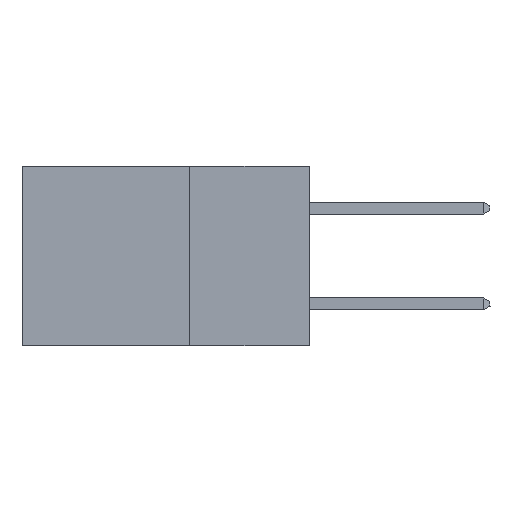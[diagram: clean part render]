
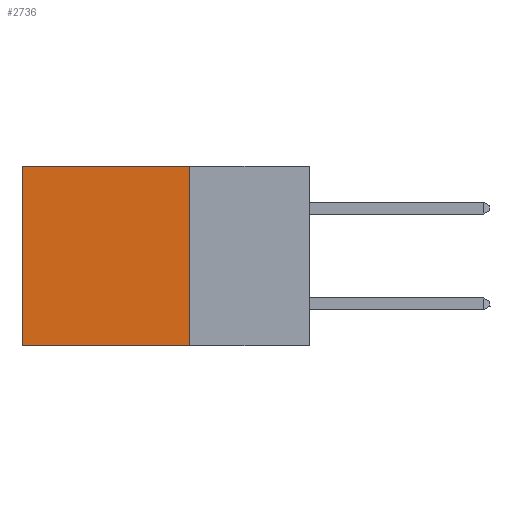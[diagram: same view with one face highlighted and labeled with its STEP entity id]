
A CAD part, left-side view. The second image highlights one B-rep face of the part: STEP entity #2736.
In plain terms, the highlighted planar face has unit normal (-1, 0, 0).
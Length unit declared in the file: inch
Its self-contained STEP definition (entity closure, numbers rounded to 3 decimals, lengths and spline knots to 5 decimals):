
#719 = ORIENTED_EDGE ( 'NONE', *, *, #4456, .T. ) ;
#1037 = EDGE_CURVE ( 'NONE', #16225, #10508, #19683, .T. ) ;
#1660 = VECTOR ( 'NONE', #12428, 39.37008 ) ;
#1872 = LINE ( 'NONE', #16064, #6905 ) ;
#2736 = ADVANCED_FACE ( 'NONE', ( #14826 ), #18105, .F. ) ;
#4456 = EDGE_CURVE ( 'NONE', #16225, #9502, #1872, .T. ) ;
#5193 = DIRECTION ( 'NONE',  ( 0., 1., 0. ) ) ;
#5533 = LINE ( 'NONE', #5628, #10541 ) ;
#5628 = CARTESIAN_POINT ( 'NONE',  ( 0.2875, 0.6, -0.375 ) ) ;
#6150 = EDGE_CURVE ( 'NONE', #9502, #11161, #5533, .T. ) ;
#6254 = ORIENTED_EDGE ( 'NONE', *, *, #1037, .F. ) ;
#6905 = VECTOR ( 'NONE', #20877, 39.37008 ) ;
#7322 = DIRECTION ( 'NONE',  ( 0., 0., -1. ) ) ;
#9097 = CARTESIAN_POINT ( 'NONE',  ( 0.2875, 0.25, 0. ) ) ;
#9502 = VERTEX_POINT ( 'NONE', #19865 ) ;
#9515 = DIRECTION ( 'NONE',  ( 0., 0., -1. ) ) ;
#10508 = VERTEX_POINT ( 'NONE', #15637 ) ;
#10541 = VECTOR ( 'NONE', #7322, 39.37008 ) ;
#10722 = CARTESIAN_POINT ( 'NONE',  ( 0.2875, 0.25, -0.375 ) ) ;
#11035 = CARTESIAN_POINT ( 'NONE',  ( 0.2875, 0.25, -0.375 ) ) ;
#11161 = VERTEX_POINT ( 'NONE', #19526 ) ;
#12034 = EDGE_CURVE ( 'NONE', #10508, #11161, #21191, .T. ) ;
#12428 = DIRECTION ( 'NONE',  ( 0., 0., -1. ) ) ;
#14046 = VECTOR ( 'NONE', #5193, 39.37008 ) ;
#14826 = FACE_OUTER_BOUND ( 'NONE', #20043, .T. ) ;
#15346 = CARTESIAN_POINT ( 'NONE',  ( 0.2875, 0.25, -0.375 ) ) ;
#15637 = CARTESIAN_POINT ( 'NONE',  ( 0.2875, 0.25, -0.375 ) ) ;
#15769 = ORIENTED_EDGE ( 'NONE', *, *, #12034, .F. ) ;
#16064 = CARTESIAN_POINT ( 'NONE',  ( 0.2875, 0.25, 0. ) ) ;
#16225 = VERTEX_POINT ( 'NONE', #9097 ) ;
#16267 = ORIENTED_EDGE ( 'NONE', *, *, #6150, .T. ) ;
#18105 = PLANE ( 'NONE',  #20484 ) ;
#19526 = CARTESIAN_POINT ( 'NONE',  ( 0.2875, 0.6, -0.375 ) ) ;
#19576 = DIRECTION ( 'NONE',  ( 1., 0., 0. ) ) ;
#19683 = LINE ( 'NONE', #10722, #1660 ) ;
#19865 = CARTESIAN_POINT ( 'NONE',  ( 0.2875, 0.6, 0. ) ) ;
#20043 = EDGE_LOOP ( 'NONE', ( #16267, #15769, #6254, #719 ) ) ;
#20484 = AXIS2_PLACEMENT_3D ( 'NONE', #11035, #19576, #9515 ) ;
#20877 = DIRECTION ( 'NONE',  ( 0., 1., 0. ) ) ;
#21191 = LINE ( 'NONE', #15346, #14046 ) ;
